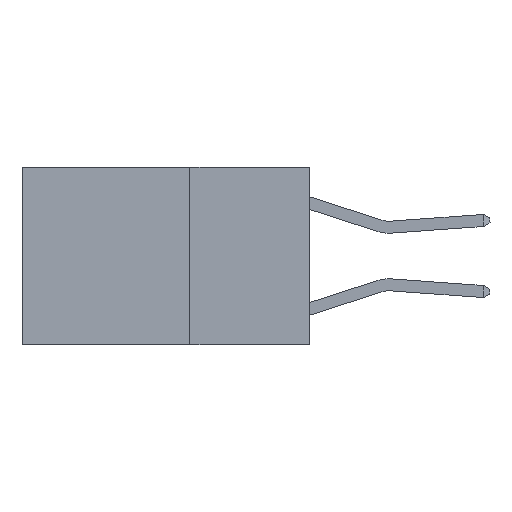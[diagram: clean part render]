
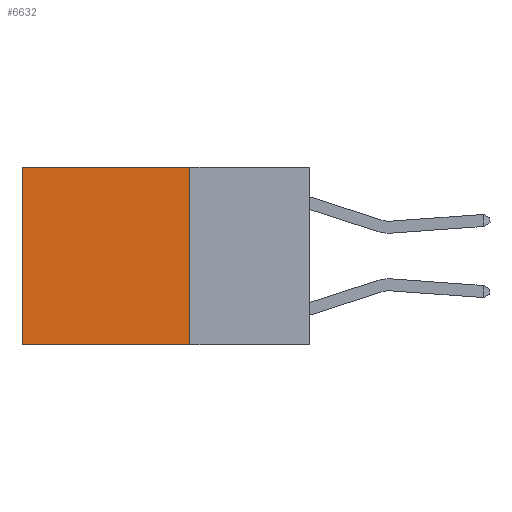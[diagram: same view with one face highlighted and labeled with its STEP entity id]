
A CAD part, left-side view. The second image highlights one B-rep face of the part: STEP entity #6632.
In plain terms, the highlighted planar face has unit normal (-1, 0, 0).
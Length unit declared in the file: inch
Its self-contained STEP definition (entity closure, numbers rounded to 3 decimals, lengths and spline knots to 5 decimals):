
#304 = DIRECTION ( 'NONE',  ( 0., 0., -1. ) ) ;
#356 = EDGE_CURVE ( 'NONE', #11688, #18328, #4208, .T. ) ;
#949 = CARTESIAN_POINT ( 'NONE',  ( 0.2625, 0.25, 0. ) ) ;
#1075 = ORIENTED_EDGE ( 'NONE', *, *, #356, .F. ) ;
#1298 = EDGE_CURVE ( 'NONE', #18554, #18616, #10730, .T. ) ;
#2426 = DIRECTION ( 'NONE',  ( 0., 0., -1. ) ) ;
#4208 = LINE ( 'NONE', #8609, #8670 ) ;
#5227 = ORIENTED_EDGE ( 'NONE', *, *, #1298, .T. ) ;
#6632 = ADVANCED_FACE ( 'NONE', ( #13825 ), #15789, .F. ) ;
#6758 = VECTOR ( 'NONE', #8035, 39.37008 ) ;
#7234 = DIRECTION ( 'NONE',  ( 0., 1., 0. ) ) ;
#7382 = CARTESIAN_POINT ( 'NONE',  ( 0.2625, 0.25, 0. ) ) ;
#7424 = EDGE_LOOP ( 'NONE', ( #11464, #1075, #17539, #5227 ) ) ;
#7657 = CARTESIAN_POINT ( 'NONE',  ( 0.2625, 0.25, 0. ) ) ;
#7882 = AXIS2_PLACEMENT_3D ( 'NONE', #949, #11380, #2426 ) ;
#8035 = DIRECTION ( 'NONE',  ( 0., 1., 0. ) ) ;
#8385 = CARTESIAN_POINT ( 'NONE',  ( 0.2625, 0.6, -0.37 ) ) ;
#8609 = CARTESIAN_POINT ( 'NONE',  ( 0.2625, 0.25, -0.37 ) ) ;
#8670 = VECTOR ( 'NONE', #7234, 39.37008 ) ;
#9729 = VECTOR ( 'NONE', #11712, 39.37008 ) ;
#10183 = EDGE_CURVE ( 'NONE', #18616, #18328, #17627, .T. ) ;
#10730 = LINE ( 'NONE', #15447, #6758 ) ;
#11380 = DIRECTION ( 'NONE',  ( 1., 0., 0. ) ) ;
#11464 = ORIENTED_EDGE ( 'NONE', *, *, #10183, .T. ) ;
#11688 = VERTEX_POINT ( 'NONE', #14101 ) ;
#11712 = DIRECTION ( 'NONE',  ( 0., 0., -1. ) ) ;
#13696 = EDGE_CURVE ( 'NONE', #18554, #11688, #19095, .T. ) ;
#13825 = FACE_OUTER_BOUND ( 'NONE', #7424, .T. ) ;
#14101 = CARTESIAN_POINT ( 'NONE',  ( 0.2625, 0.25, -0.37 ) ) ;
#14700 = CARTESIAN_POINT ( 'NONE',  ( 0.2625, 0.6, 0. ) ) ;
#15171 = VECTOR ( 'NONE', #304, 39.37008 ) ;
#15447 = CARTESIAN_POINT ( 'NONE',  ( 0.2625, 0.25, 0. ) ) ;
#15789 = PLANE ( 'NONE',  #7882 ) ;
#16433 = CARTESIAN_POINT ( 'NONE',  ( 0.2625, 0.6, 0. ) ) ;
#17539 = ORIENTED_EDGE ( 'NONE', *, *, #13696, .F. ) ;
#17627 = LINE ( 'NONE', #14700, #9729 ) ;
#18328 = VERTEX_POINT ( 'NONE', #8385 ) ;
#18554 = VERTEX_POINT ( 'NONE', #7382 ) ;
#18616 = VERTEX_POINT ( 'NONE', #16433 ) ;
#19095 = LINE ( 'NONE', #7657, #15171 ) ;
